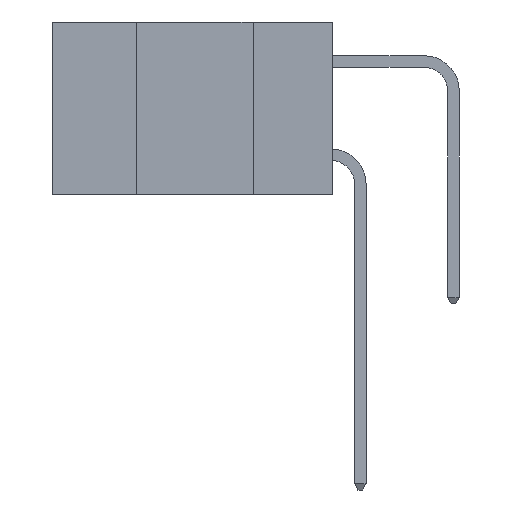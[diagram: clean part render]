
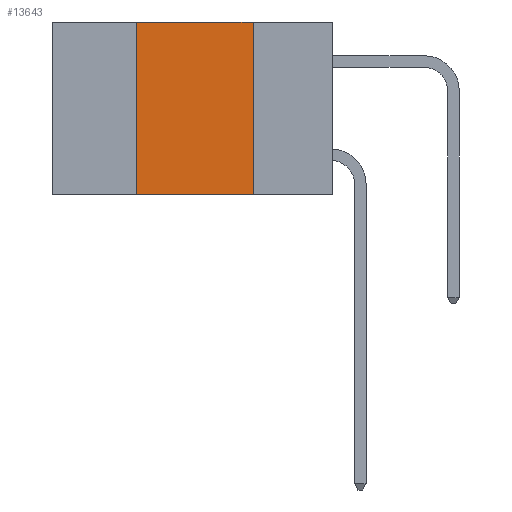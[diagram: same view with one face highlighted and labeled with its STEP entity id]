
A CAD part, left-side view. The second image highlights one B-rep face of the part: STEP entity #13643.
In plain terms, the highlighted planar face has unit normal (-1, 0, 0).
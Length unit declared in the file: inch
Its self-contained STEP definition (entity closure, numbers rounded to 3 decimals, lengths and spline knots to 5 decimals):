
#1385 = AXIS2_PLACEMENT_3D ( 'NONE', #9957, #2076, #11211 ) ;
#2076 = DIRECTION ( 'NONE',  ( 1., 0., 0. ) ) ;
#2461 = LINE ( 'NONE', #3924, #9058 ) ;
#2539 = CARTESIAN_POINT ( 'NONE',  ( 0., 0.17, -0.37 ) ) ;
#2566 = LINE ( 'NONE', #4645, #12493 ) ;
#2897 = LINE ( 'NONE', #5077, #16551 ) ;
#2928 = LINE ( 'NONE', #10362, #13263 ) ;
#3027 = EDGE_CURVE ( 'NONE', #16560, #15768, #2566, .T. ) ;
#3902 = EDGE_CURVE ( 'NONE', #16560, #13937, #2928, .T. ) ;
#3924 = CARTESIAN_POINT ( 'NONE',  ( 0., 0.17, -0.37 ) ) ;
#3986 = DIRECTION ( 'NONE',  ( 0., 0., -1. ) ) ;
#4645 = CARTESIAN_POINT ( 'NONE',  ( 0., 0.6, -0.37 ) ) ;
#4764 = EDGE_CURVE ( 'NONE', #13937, #13672, #2897, .T. ) ;
#5077 = CARTESIAN_POINT ( 'NONE',  ( 0., 0.6, 0. ) ) ;
#5659 = EDGE_CURVE ( 'NONE', #13672, #15768, #2461, .T. ) ;
#5920 = ORIENTED_EDGE ( 'NONE', *, *, #5659, .F. ) ;
#5977 = PLANE ( 'NONE',  #1385 ) ;
#6070 = DIRECTION ( 'NONE',  ( 0., -1., 0. ) ) ;
#6952 = ORIENTED_EDGE ( 'NONE', *, *, #4764, .F. ) ;
#8079 = EDGE_LOOP ( 'NONE', ( #5920, #6952, #13812, #10320 ) ) ;
#9058 = VECTOR ( 'NONE', #3986, 39.37008 ) ;
#9642 = DIRECTION ( 'NONE',  ( 0., -1., 0. ) ) ;
#9957 = CARTESIAN_POINT ( 'NONE',  ( 0., 0.6, 0. ) ) ;
#10320 = ORIENTED_EDGE ( 'NONE', *, *, #3027, .T. ) ;
#10362 = CARTESIAN_POINT ( 'NONE',  ( 0., 0.42, -0.37 ) ) ;
#10934 = DIRECTION ( 'NONE',  ( 0., 0., 1. ) ) ;
#11211 = DIRECTION ( 'NONE',  ( 0., 0., -1. ) ) ;
#11265 = CARTESIAN_POINT ( 'NONE',  ( 0., 0.17, 0. ) ) ;
#12493 = VECTOR ( 'NONE', #9642, 39.37008 ) ;
#13263 = VECTOR ( 'NONE', #10934, 39.37008 ) ;
#13643 = ADVANCED_FACE ( 'NONE', ( #14339 ), #5977, .F. ) ;
#13672 = VERTEX_POINT ( 'NONE', #11265 ) ;
#13725 = CARTESIAN_POINT ( 'NONE',  ( 0., 0.42, 0. ) ) ;
#13812 = ORIENTED_EDGE ( 'NONE', *, *, #3902, .F. ) ;
#13937 = VERTEX_POINT ( 'NONE', #13725 ) ;
#14339 = FACE_OUTER_BOUND ( 'NONE', #8079, .T. ) ;
#15750 = CARTESIAN_POINT ( 'NONE',  ( 0., 0.42, -0.37 ) ) ;
#15768 = VERTEX_POINT ( 'NONE', #2539 ) ;
#16551 = VECTOR ( 'NONE', #6070, 39.37008 ) ;
#16560 = VERTEX_POINT ( 'NONE', #15750 ) ;
